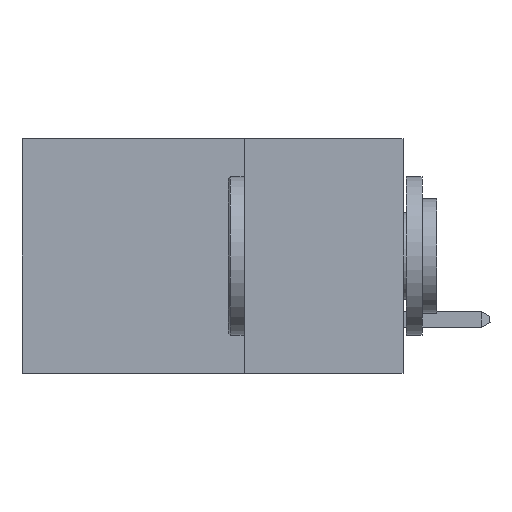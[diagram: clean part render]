
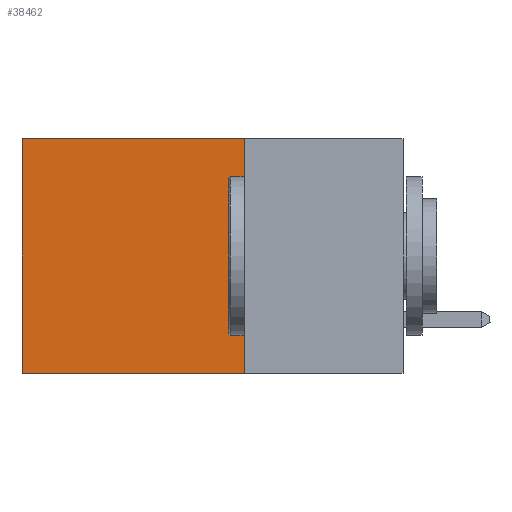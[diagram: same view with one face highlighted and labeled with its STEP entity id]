
A CAD part, left-side view. The second image highlights one B-rep face of the part: STEP entity #38462.
In plain terms, the highlighted planar face has unit normal (-1, 0, 0).
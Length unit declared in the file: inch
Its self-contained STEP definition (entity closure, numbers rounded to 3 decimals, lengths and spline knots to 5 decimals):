
#302 = DIRECTION ( 'NONE',  ( 1., 0., 0. ) ) ;
#1470 = DIRECTION ( 'NONE',  ( 0., 1., 0. ) ) ;
#2024 = ORIENTED_EDGE ( 'NONE', *, *, #5107, .T. ) ;
#3621 = CARTESIAN_POINT ( 'NONE',  ( 0.2875, 0.25, 0. ) ) ;
#5107 = EDGE_CURVE ( 'NONE', #6389, #25902, #36387, .T. ) ;
#5678 = DIRECTION ( 'NONE',  ( 0., 0., -1. ) ) ;
#6389 = VERTEX_POINT ( 'NONE', #3621 ) ;
#6713 = ORIENTED_EDGE ( 'NONE', *, *, #26288, .F. ) ;
#8299 = EDGE_LOOP ( 'NONE', ( #16131, #13908, #6713, #2024 ) ) ;
#9374 = VERTEX_POINT ( 'NONE', #30911 ) ;
#11201 = LINE ( 'NONE', #35771, #32978 ) ;
#11335 = VECTOR ( 'NONE', #1470, 39.37008 ) ;
#12164 = CARTESIAN_POINT ( 'NONE',  ( 0.2875, 0.25, 0. ) ) ;
#12609 = EDGE_CURVE ( 'NONE', #25902, #9374, #11201, .T. ) ;
#12768 = CARTESIAN_POINT ( 'NONE',  ( 0.2875, 0.25, -0.37 ) ) ;
#13908 = ORIENTED_EDGE ( 'NONE', *, *, #31931, .F. ) ;
#14112 = FACE_OUTER_BOUND ( 'NONE', #8299, .T. ) ;
#15076 = VERTEX_POINT ( 'NONE', #12768 ) ;
#15678 = CARTESIAN_POINT ( 'NONE',  ( 0.2875, 0.6, 0. ) ) ;
#16131 = ORIENTED_EDGE ( 'NONE', *, *, #12609, .T. ) ;
#18108 = PLANE ( 'NONE',  #33649 ) ;
#20366 = LINE ( 'NONE', #20480, #35216 ) ;
#20480 = CARTESIAN_POINT ( 'NONE',  ( 0.2875, 0.25, 0. ) ) ;
#20992 = DIRECTION ( 'NONE',  ( 0., 0., -1. ) ) ;
#21099 = DIRECTION ( 'NONE',  ( 0., 0., -1. ) ) ;
#22978 = CARTESIAN_POINT ( 'NONE',  ( 0.2875, 0.25, 0. ) ) ;
#25902 = VERTEX_POINT ( 'NONE', #15678 ) ;
#25965 = DIRECTION ( 'NONE',  ( 0., 1., 0. ) ) ;
#26288 = EDGE_CURVE ( 'NONE', #6389, #15076, #20366, .T. ) ;
#28532 = VECTOR ( 'NONE', #25965, 39.37008 ) ;
#30911 = CARTESIAN_POINT ( 'NONE',  ( 0.2875, 0.6, -0.37 ) ) ;
#31067 = CARTESIAN_POINT ( 'NONE',  ( 0.2875, 0.25, -0.37 ) ) ;
#31931 = EDGE_CURVE ( 'NONE', #15076, #9374, #35906, .T. ) ;
#32978 = VECTOR ( 'NONE', #20992, 39.37008 ) ;
#33649 = AXIS2_PLACEMENT_3D ( 'NONE', #12164, #302, #21099 ) ;
#35216 = VECTOR ( 'NONE', #5678, 39.37008 ) ;
#35771 = CARTESIAN_POINT ( 'NONE',  ( 0.2875, 0.6, 0. ) ) ;
#35906 = LINE ( 'NONE', #31067, #11335 ) ;
#36387 = LINE ( 'NONE', #22978, #28532 ) ;
#38462 = ADVANCED_FACE ( 'NONE', ( #14112 ), #18108, .F. ) ;
